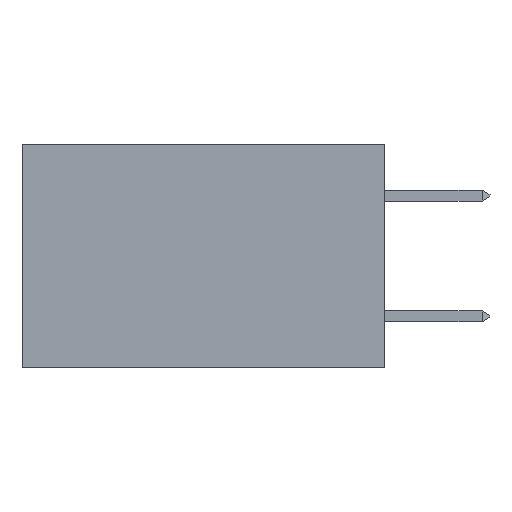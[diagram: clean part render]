
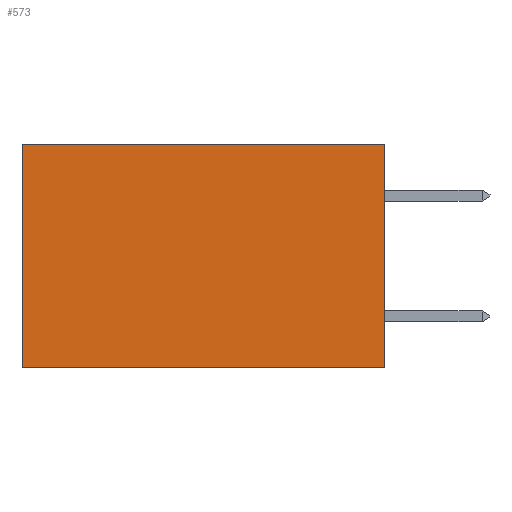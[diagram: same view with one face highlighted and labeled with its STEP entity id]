
A CAD part, left-side view. The second image highlights one B-rep face of the part: STEP entity #573.
In plain terms, the highlighted planar face has unit normal (-1, 0, 0).
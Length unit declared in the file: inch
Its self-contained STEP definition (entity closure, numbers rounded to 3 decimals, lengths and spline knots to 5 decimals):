
#542 = DIRECTION ( 'NONE',  ( 0., 0., -1. ) ) ;
#573 = ADVANCED_FACE ( 'NONE', ( #4615 ), #4297, .F. ) ;
#944 = EDGE_CURVE ( 'NONE', #1222, #3894, #5077, .T. ) ;
#990 = CARTESIAN_POINT ( 'NONE',  ( 0.2875, 0.6, -0.37 ) ) ;
#1222 = VERTEX_POINT ( 'NONE', #12026 ) ;
#2471 = LINE ( 'NONE', #4025, #10000 ) ;
#2924 = VECTOR ( 'NONE', #542, 39.37008 ) ;
#3354 = VECTOR ( 'NONE', #5502, 39.37008 ) ;
#3617 = ORIENTED_EDGE ( 'NONE', *, *, #944, .F. ) ;
#3723 = ORIENTED_EDGE ( 'NONE', *, *, #12434, .T. ) ;
#3894 = VERTEX_POINT ( 'NONE', #990 ) ;
#4025 = CARTESIAN_POINT ( 'NONE',  ( 0.2875, 0., 0. ) ) ;
#4153 = DIRECTION ( 'NONE',  ( 0., 1., 0. ) ) ;
#4204 = EDGE_CURVE ( 'NONE', #12014, #8056, #2471, .T. ) ;
#4242 = DIRECTION ( 'NONE',  ( 0., 0., -1. ) ) ;
#4258 = DIRECTION ( 'NONE',  ( 1., 0., 0. ) ) ;
#4297 = PLANE ( 'NONE',  #10331 ) ;
#4350 = ORIENTED_EDGE ( 'NONE', *, *, #4204, .T. ) ;
#4370 = ORIENTED_EDGE ( 'NONE', *, *, #11935, .F. ) ;
#4395 = CARTESIAN_POINT ( 'NONE',  ( 0.2875, 0., 0. ) ) ;
#4615 = FACE_OUTER_BOUND ( 'NONE', #10560, .T. ) ;
#4840 = DIRECTION ( 'NONE',  ( 0., 0., -1. ) ) ;
#4956 = VECTOR ( 'NONE', #4840, 39.37008 ) ;
#5077 = LINE ( 'NONE', #7713, #3354 ) ;
#5265 = LINE ( 'NONE', #10696, #4956 ) ;
#5502 = DIRECTION ( 'NONE',  ( 0., 1., 0. ) ) ;
#5573 = LINE ( 'NONE', #11291, #2924 ) ;
#7713 = CARTESIAN_POINT ( 'NONE',  ( 0.2875, 0., -0.37 ) ) ;
#8056 = VERTEX_POINT ( 'NONE', #11894 ) ;
#9765 = CARTESIAN_POINT ( 'NONE',  ( 0.2875, 0., 0. ) ) ;
#10000 = VECTOR ( 'NONE', #4153, 39.37008 ) ;
#10331 = AXIS2_PLACEMENT_3D ( 'NONE', #4395, #4258, #4242 ) ;
#10560 = EDGE_LOOP ( 'NONE', ( #3723, #3617, #4370, #4350 ) ) ;
#10696 = CARTESIAN_POINT ( 'NONE',  ( 0.2875, 0., 0. ) ) ;
#11291 = CARTESIAN_POINT ( 'NONE',  ( 0.2875, 0.6, 0. ) ) ;
#11894 = CARTESIAN_POINT ( 'NONE',  ( 0.2875, 0.6, 0. ) ) ;
#11935 = EDGE_CURVE ( 'NONE', #12014, #1222, #5265, .T. ) ;
#12014 = VERTEX_POINT ( 'NONE', #9765 ) ;
#12026 = CARTESIAN_POINT ( 'NONE',  ( 0.2875, 0., -0.37 ) ) ;
#12434 = EDGE_CURVE ( 'NONE', #8056, #3894, #5573, .T. ) ;
